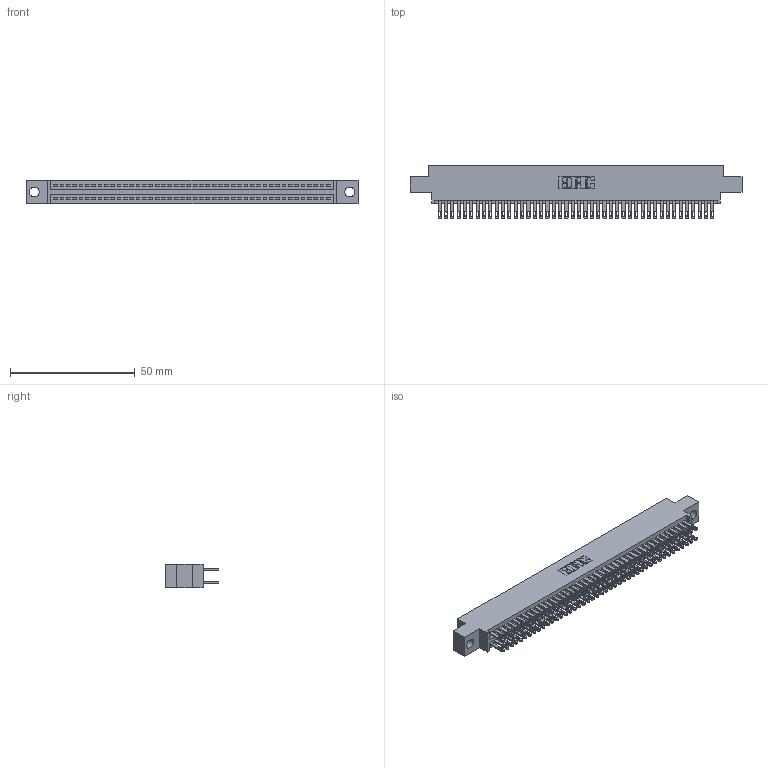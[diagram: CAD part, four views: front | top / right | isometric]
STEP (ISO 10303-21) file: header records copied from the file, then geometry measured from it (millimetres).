
FILE_DESCRIPTION (( 'STEP AP203' ), '1' );
FILE_NAME ('345-088-500-804.STEP', '2021-05-20T13:52:30', ( '' ), ( '' ), 'SwSTEP 2.0', 'SolidWorks 2020', '' );
FILE_SCHEMA (( 'CONFIG_CONTROL_DESIGN' ));
Length unit declared in the file: inch
Products named in the file (3): 345-292-001_345-293-100; 345 Part_0.170 Offset - 0.156 Dia-TI; 345-088-500-804
Assembly tree (89 placements, depth 2):
  345-088-500-804
    345 Part_0.170 Offset - 0.156 Dia-TI
    345-292-001_345-293-100  x88
Bounding box: 132.97 x 21.51 x 9.4 mm (x, y, z)
Volume: 12984.9 mm3; surface area: 20125.2 mm2
Topology: 89 solids, 89 shells, 4192 faces, 12797 edges, 8530 vertices
Faces by surface type: plane 2474, cylinder 1718
Entity records: 34735 total; most frequent: CARTESIAN_POINT 5826, ORIENTED_EDGE 5758, DIRECTION 5135, EDGE_CURVE 2879, LINE 2567, VECTOR 2567, VERTEX_POINT 1918, AXIS2_PLACEMENT_3D 1284
